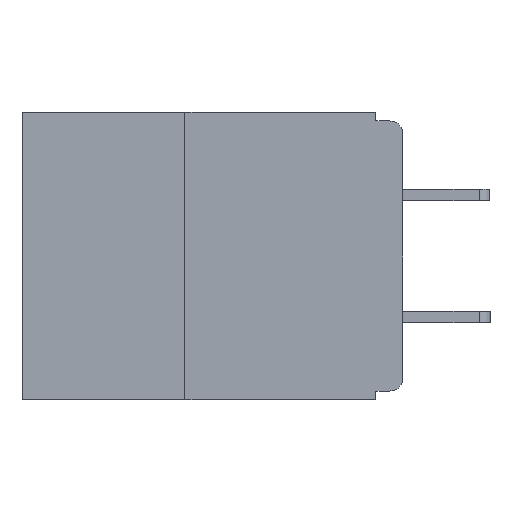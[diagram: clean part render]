
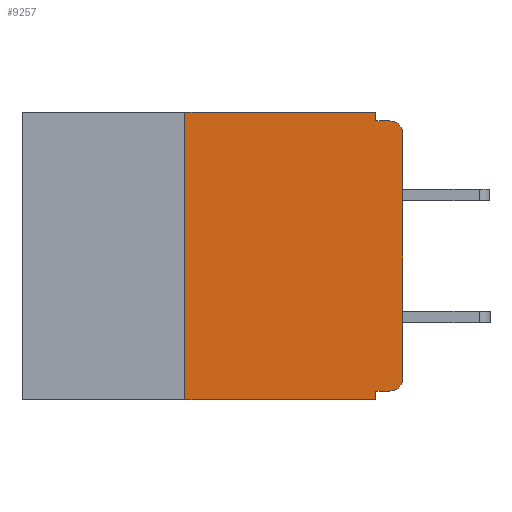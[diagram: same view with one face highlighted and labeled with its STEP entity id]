
A CAD part, left-side view. The second image highlights one B-rep face of the part: STEP entity #9257.
In plain terms, the highlighted planar face has unit normal (-1, 0, 0).
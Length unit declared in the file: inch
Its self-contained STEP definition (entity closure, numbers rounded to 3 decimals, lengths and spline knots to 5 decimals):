
#160 = EDGE_CURVE ( 'NONE', #7013, #7012, #6928, .T. ) ;
#171 = VERTEX_POINT ( 'NONE', #15802 ) ;
#191 = VERTEX_POINT ( 'NONE', #2371 ) ;
#338 = DIRECTION ( 'NONE',  ( 0., -1., 0. ) ) ;
#496 = ORIENTED_EDGE ( 'NONE', *, *, #23801, .T. ) ;
#680 = CARTESIAN_POINT ( 'NONE',  ( 0., 0.437, -0.33 ) ) ;
#1470 = CARTESIAN_POINT ( 'NONE',  ( 0., 0., -0.01 ) ) ;
#1840 = LINE ( 'NONE', #680, #21058 ) ;
#1870 = EDGE_CURVE ( 'NONE', #3580, #7012, #1840, .T. ) ;
#2257 = ORIENTED_EDGE ( 'NONE', *, *, #160, .F. ) ;
#2289 = EDGE_CURVE ( 'NONE', #2329, #191, #17379, .T. ) ;
#2329 = VERTEX_POINT ( 'NONE', #18913 ) ;
#2371 = CARTESIAN_POINT ( 'NONE',  ( 0., 0., -0.305 ) ) ;
#2583 = CARTESIAN_POINT ( 'NONE',  ( 0., 0.015, -0.01 ) ) ;
#3128 = DIRECTION ( 'NONE',  ( 0., 0., -1. ) ) ;
#3150 = CARTESIAN_POINT ( 'NONE',  ( 0., 0.031, 0. ) ) ;
#3239 = EDGE_CURVE ( 'NONE', #16357, #12566, #10109, .T. ) ;
#3468 = ORIENTED_EDGE ( 'NONE', *, *, #6194, .T. ) ;
#3570 = EDGE_CURVE ( 'NONE', #3580, #16357, #17581, .T. ) ;
#3580 = VERTEX_POINT ( 'NONE', #4304 ) ;
#3587 = VECTOR ( 'NONE', #18345, 39.37008 ) ;
#3693 = EDGE_CURVE ( 'NONE', #12566, #171, #10363, .T. ) ;
#3708 = ORIENTED_EDGE ( 'NONE', *, *, #11315, .F. ) ;
#3946 = LINE ( 'NONE', #22478, #4550 ) ;
#4304 = CARTESIAN_POINT ( 'NONE',  ( 0., 0.25, -0.33 ) ) ;
#4492 = DIRECTION ( 'NONE',  ( 0., 0., 1. ) ) ;
#4501 = AXIS2_PLACEMENT_3D ( 'NONE', #23736, #7279, #20256 ) ;
#4507 = ORIENTED_EDGE ( 'NONE', *, *, #3570, .F. ) ;
#4550 = VECTOR ( 'NONE', #17152, 39.37008 ) ;
#4556 = CARTESIAN_POINT ( 'NONE',  ( 0., 0.25, -0.33 ) ) ;
#4686 = VECTOR ( 'NONE', #3128, 39.37008 ) ;
#4854 = ORIENTED_EDGE ( 'NONE', *, *, #15906, .F. ) ;
#6194 = EDGE_CURVE ( 'NONE', #191, #16907, #23894, .T. ) ;
#6255 = DIRECTION ( 'NONE',  ( 0., 0., -1. ) ) ;
#6928 = LINE ( 'NONE', #15770, #21098 ) ;
#6991 = CARTESIAN_POINT ( 'NONE',  ( 0., 0., 0. ) ) ;
#7012 = VERTEX_POINT ( 'NONE', #22170 ) ;
#7013 = VERTEX_POINT ( 'NONE', #23970 ) ;
#7279 = DIRECTION ( 'NONE',  ( 1., 0., 0. ) ) ;
#7538 = ORIENTED_EDGE ( 'NONE', *, *, #1870, .T. ) ;
#7657 = VECTOR ( 'NONE', #4492, 39.37008 ) ;
#7861 = EDGE_LOOP ( 'NONE', ( #3468, #496, #4854, #10934, #16562, #4507, #7538, #2257, #3708, #13619 ) ) ;
#8494 = DIRECTION ( 'NONE',  ( 0., -1., 0. ) ) ;
#8544 = CARTESIAN_POINT ( 'NONE',  ( 0., 0.437, 0. ) ) ;
#8639 = CARTESIAN_POINT ( 'NONE',  ( 0., 0.015, -0.025 ) ) ;
#9257 = ADVANCED_FACE ( 'NONE', ( #18694 ), #18437, .F. ) ;
#10109 = LINE ( 'NONE', #8544, #19322 ) ;
#10363 = LINE ( 'NONE', #3150, #4686 ) ;
#10564 = DIRECTION ( 'NONE',  ( 0., 0., -1. ) ) ;
#10934 = ORIENTED_EDGE ( 'NONE', *, *, #3693, .F. ) ;
#11315 = EDGE_CURVE ( 'NONE', #2329, #7013, #3946, .T. ) ;
#12188 = CIRCLE ( 'NONE', #15737, 0.015 ) ;
#12566 = VERTEX_POINT ( 'NONE', #19015 ) ;
#12724 = VERTEX_POINT ( 'NONE', #2583 ) ;
#13619 = ORIENTED_EDGE ( 'NONE', *, *, #2289, .T. ) ;
#14265 = CARTESIAN_POINT ( 'NONE',  ( 0., 0.25, 0. ) ) ;
#15737 = AXIS2_PLACEMENT_3D ( 'NONE', #8639, #21506, #10564 ) ;
#15753 = CARTESIAN_POINT ( 'NONE',  ( 0., 0., -0.025 ) ) ;
#15770 = CARTESIAN_POINT ( 'NONE',  ( 0., 0.031, -0.33 ) ) ;
#15802 = CARTESIAN_POINT ( 'NONE',  ( 0., 0.031, -0.01 ) ) ;
#15906 = EDGE_CURVE ( 'NONE', #171, #12724, #18528, .T. ) ;
#16357 = VERTEX_POINT ( 'NONE', #14265 ) ;
#16562 = ORIENTED_EDGE ( 'NONE', *, *, #3239, .F. ) ;
#16907 = VERTEX_POINT ( 'NONE', #15753 ) ;
#17152 = DIRECTION ( 'NONE',  ( 0., 1., 0. ) ) ;
#17379 = CIRCLE ( 'NONE', #17878, 0.015 ) ;
#17581 = LINE ( 'NONE', #4556, #7657 ) ;
#17878 = AXIS2_PLACEMENT_3D ( 'NONE', #19292, #19278, #19271 ) ;
#18345 = DIRECTION ( 'NONE',  ( 0., -1., 0. ) ) ;
#18437 = PLANE ( 'NONE',  #4501 ) ;
#18528 = LINE ( 'NONE', #1470, #3587 ) ;
#18599 = VECTOR ( 'NONE', #19995, 39.37008 ) ;
#18694 = FACE_OUTER_BOUND ( 'NONE', #7861, .T. ) ;
#18913 = CARTESIAN_POINT ( 'NONE',  ( 0., 0.015, -0.32 ) ) ;
#19015 = CARTESIAN_POINT ( 'NONE',  ( 0., 0.031, 0. ) ) ;
#19271 = DIRECTION ( 'NONE',  ( 0., 0., -1. ) ) ;
#19278 = DIRECTION ( 'NONE',  ( -1., 0., 0. ) ) ;
#19292 = CARTESIAN_POINT ( 'NONE',  ( 0., 0.015, -0.305 ) ) ;
#19322 = VECTOR ( 'NONE', #8494, 39.37008 ) ;
#19995 = DIRECTION ( 'NONE',  ( 0., 0., 1. ) ) ;
#20256 = DIRECTION ( 'NONE',  ( 0., 0., -1. ) ) ;
#21058 = VECTOR ( 'NONE', #338, 39.37008 ) ;
#21098 = VECTOR ( 'NONE', #6255, 39.37008 ) ;
#21506 = DIRECTION ( 'NONE',  ( -1., 0., 0. ) ) ;
#22170 = CARTESIAN_POINT ( 'NONE',  ( 0., 0.031, -0.33 ) ) ;
#22478 = CARTESIAN_POINT ( 'NONE',  ( 0., 0., -0.32 ) ) ;
#23736 = CARTESIAN_POINT ( 'NONE',  ( 0., 0.437, 0. ) ) ;
#23801 = EDGE_CURVE ( 'NONE', #16907, #12724, #12188, .T. ) ;
#23894 = LINE ( 'NONE', #6991, #18599 ) ;
#23970 = CARTESIAN_POINT ( 'NONE',  ( 0., 0.031, -0.32 ) ) ;
